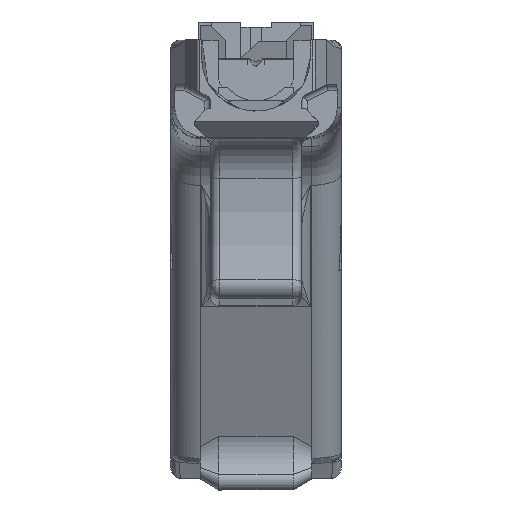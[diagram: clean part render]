
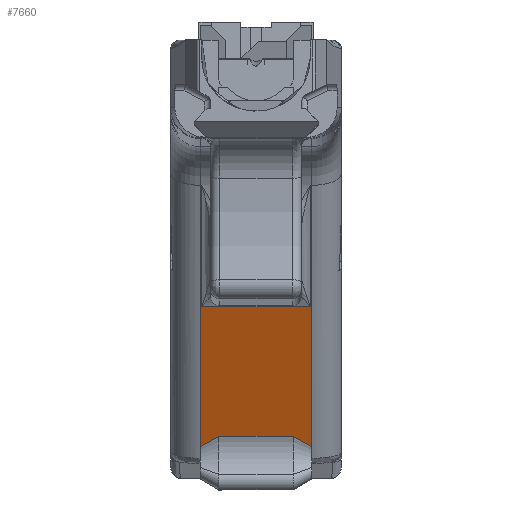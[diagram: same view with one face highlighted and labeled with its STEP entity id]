
A CAD part, top view. The second image highlights one B-rep face of the part: STEP entity #7660.
In plain terms, the highlighted planar face has unit normal (0, -0.407, 0.914).
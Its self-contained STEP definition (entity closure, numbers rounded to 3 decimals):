
#395=FACE_OUTER_BOUND('',#815,.T.);
#815=EDGE_LOOP('',(#5525,#5526,#5527,#5528,#5529,#5530,#5531,#5532,#5533,
#5534));
#1620=LINE('',#12314,#2391);
#1621=LINE('',#12316,#2392);
#1622=LINE('',#12318,#2393);
#1623=LINE('',#12320,#2394);
#1624=LINE('',#12322,#2395);
#1625=LINE('',#12324,#2396);
#1626=LINE('',#12326,#2397);
#1627=LINE('',#12328,#2398);
#1628=LINE('',#12330,#2399);
#1629=LINE('',#12331,#2400);
#2391=VECTOR('',#9326,1000.);
#2392=VECTOR('',#9327,1000.);
#2393=VECTOR('',#9328,1000.);
#2394=VECTOR('',#9329,1000.);
#2395=VECTOR('',#9330,1000.);
#2396=VECTOR('',#9331,1000.);
#2397=VECTOR('',#9332,1000.);
#2398=VECTOR('',#9333,1000.);
#2399=VECTOR('',#9334,1000.);
#2400=VECTOR('',#9335,1000.);
#3344=VERTEX_POINT('',#12312);
#3345=VERTEX_POINT('',#12313);
#3346=VERTEX_POINT('',#12315);
#3347=VERTEX_POINT('',#12317);
#3348=VERTEX_POINT('',#12319);
#3349=VERTEX_POINT('',#12321);
#3350=VERTEX_POINT('',#12323);
#3351=VERTEX_POINT('',#12325);
#3352=VERTEX_POINT('',#12327);
#3353=VERTEX_POINT('',#12329);
#4183=EDGE_CURVE('',#3344,#3345,#1620,.T.);
#4184=EDGE_CURVE('',#3346,#3344,#1621,.T.);
#4185=EDGE_CURVE('',#3347,#3346,#1622,.T.);
#4186=EDGE_CURVE('',#3347,#3348,#1623,.T.);
#4187=EDGE_CURVE('',#3348,#3349,#1624,.T.);
#4188=EDGE_CURVE('',#3349,#3350,#1625,.T.);
#4189=EDGE_CURVE('',#3350,#3351,#1626,.T.);
#4190=EDGE_CURVE('',#3351,#3352,#1627,.T.);
#4191=EDGE_CURVE('',#3352,#3353,#1628,.T.);
#4192=EDGE_CURVE('',#3353,#3345,#1629,.T.);
#5525=ORIENTED_EDGE('',*,*,#4183,.F.);
#5526=ORIENTED_EDGE('',*,*,#4184,.F.);
#5527=ORIENTED_EDGE('',*,*,#4185,.F.);
#5528=ORIENTED_EDGE('',*,*,#4186,.T.);
#5529=ORIENTED_EDGE('',*,*,#4187,.T.);
#5530=ORIENTED_EDGE('',*,*,#4188,.T.);
#5531=ORIENTED_EDGE('',*,*,#4189,.T.);
#5532=ORIENTED_EDGE('',*,*,#4190,.T.);
#5533=ORIENTED_EDGE('',*,*,#4191,.T.);
#5534=ORIENTED_EDGE('',*,*,#4192,.T.);
#7384=PLANE('',#8197);
#7660=ADVANCED_FACE('',(#395),#7384,.F.);
#8197=AXIS2_PLACEMENT_3D('',#12311,#9324,#9325);
#9324=DIRECTION('center_axis',(0.,0.407,-0.914));
#9325=DIRECTION('ref_axis',(0.,0.914,0.407));
#9326=DIRECTION('',(-0.857,-0.471,-0.21));
#9327=DIRECTION('',(-1.,0.,0.));
#9328=DIRECTION('',(-0.857,0.471,0.21));
#9329=DIRECTION('',(0.,0.914,0.407));
#9330=DIRECTION('',(-1.,0.,0.));
#9331=DIRECTION('',(0.,-0.914,-0.407));
#9332=DIRECTION('',(-1.,0.,0.));
#9333=DIRECTION('',(0.,0.914,0.407));
#9334=DIRECTION('',(-1.,0.,0.));
#9335=DIRECTION('',(0.,-0.914,-0.407));
#12311=CARTESIAN_POINT('Origin',(14.605,-24.741,-86.105));
#12312=CARTESIAN_POINT('',(-6.35,-67.661,-105.21));
#12313=CARTESIAN_POINT('',(-9.525,-69.405,-105.986));
#12314=CARTESIAN_POINT('',(-7.938,-68.533,-105.598));
#12315=CARTESIAN_POINT('',(6.35,-67.661,-105.21));
#12316=CARTESIAN_POINT('',(6.35,-67.661,-105.21));
#12317=CARTESIAN_POINT('',(9.525,-69.405,-105.986));
#12318=CARTESIAN_POINT('',(7.938,-68.533,-105.598));
#12319=CARTESIAN_POINT('',(9.525,-24.741,-86.105));
#12320=CARTESIAN_POINT('',(9.525,-24.741,-86.105));
#12321=CARTESIAN_POINT('',(9.271,-24.741,-86.105));
#12322=CARTESIAN_POINT('',(14.605,-24.741,-86.105));
#12323=CARTESIAN_POINT('',(9.271,-45.529,-95.358));
#12324=CARTESIAN_POINT('',(9.271,-24.741,-86.105));
#12325=CARTESIAN_POINT('',(-9.271,-45.529,-95.358));
#12326=CARTESIAN_POINT('',(7.747,-45.529,-95.358));
#12327=CARTESIAN_POINT('',(-9.271,-24.741,-86.105));
#12328=CARTESIAN_POINT('',(-9.271,-24.741,-86.105));
#12329=CARTESIAN_POINT('',(-9.525,-24.741,-86.105));
#12330=CARTESIAN_POINT('',(14.605,-24.741,-86.105));
#12331=CARTESIAN_POINT('',(-9.525,-24.741,-86.105));
